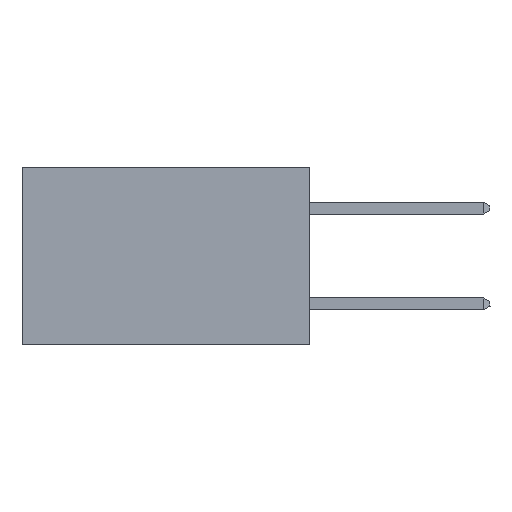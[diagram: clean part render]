
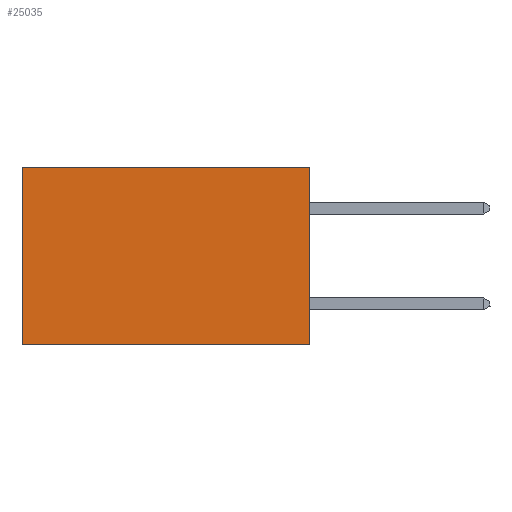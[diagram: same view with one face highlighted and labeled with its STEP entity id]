
A CAD part, left-side view. The second image highlights one B-rep face of the part: STEP entity #25035.
In plain terms, the highlighted planar face has unit normal (-1, 0, 0).
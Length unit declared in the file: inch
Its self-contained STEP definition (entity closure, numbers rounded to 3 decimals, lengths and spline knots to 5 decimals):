
#95 = EDGE_CURVE ( 'NONE', #11923, #24437, #12233, .T. ) ;
#900 = DIRECTION ( 'NONE',  ( 0., 1., 0. ) ) ;
#1596 = DIRECTION ( 'NONE',  ( 0., 0., -1. ) ) ;
#2144 = VECTOR ( 'NONE', #900, 39.37008 ) ;
#4816 = EDGE_CURVE ( 'NONE', #11923, #17204, #19692, .T. ) ;
#5724 = CARTESIAN_POINT ( 'NONE',  ( 0.2875, 0., 0. ) ) ;
#6483 = CARTESIAN_POINT ( 'NONE',  ( 0.2875, 0.6, 0. ) ) ;
#7051 = CARTESIAN_POINT ( 'NONE',  ( 0.2875, 0.6, 0. ) ) ;
#8110 = VECTOR ( 'NONE', #15023, 39.37008 ) ;
#8834 = VECTOR ( 'NONE', #14239, 39.37008 ) ;
#10736 = CARTESIAN_POINT ( 'NONE',  ( 0.2875, 0., 0. ) ) ;
#11923 = VERTEX_POINT ( 'NONE', #12074 ) ;
#12074 = CARTESIAN_POINT ( 'NONE',  ( 0.2875, 0., 0. ) ) ;
#12233 = LINE ( 'NONE', #5724, #8110 ) ;
#13004 = DIRECTION ( 'NONE',  ( 1., 0., 0. ) ) ;
#13359 = EDGE_CURVE ( 'NONE', #17204, #30338, #27809, .T. ) ;
#13988 = ORIENTED_EDGE ( 'NONE', *, *, #95, .F. ) ;
#14239 = DIRECTION ( 'NONE',  ( 0., 0., -1. ) ) ;
#14667 = EDGE_CURVE ( 'NONE', #24437, #30338, #15170, .T. ) ;
#15023 = DIRECTION ( 'NONE',  ( 0., 0., -1. ) ) ;
#15170 = LINE ( 'NONE', #23487, #19261 ) ;
#17100 = CARTESIAN_POINT ( 'NONE',  ( 0.2875, 0.6, -0.37 ) ) ;
#17204 = VERTEX_POINT ( 'NONE', #6483 ) ;
#18708 = ORIENTED_EDGE ( 'NONE', *, *, #4816, .T. ) ;
#19261 = VECTOR ( 'NONE', #25589, 39.37008 ) ;
#19692 = LINE ( 'NONE', #10736, #2144 ) ;
#20049 = CARTESIAN_POINT ( 'NONE',  ( 0.2875, 0., 0. ) ) ;
#21058 = AXIS2_PLACEMENT_3D ( 'NONE', #20049, #13004, #1596 ) ;
#22108 = PLANE ( 'NONE',  #21058 ) ;
#23107 = EDGE_LOOP ( 'NONE', ( #28930, #25601, #13988, #18708 ) ) ;
#23365 = CARTESIAN_POINT ( 'NONE',  ( 0.2875, 0., -0.37 ) ) ;
#23487 = CARTESIAN_POINT ( 'NONE',  ( 0.2875, 0., -0.37 ) ) ;
#24437 = VERTEX_POINT ( 'NONE', #23365 ) ;
#25035 = ADVANCED_FACE ( 'NONE', ( #26280 ), #22108, .F. ) ;
#25589 = DIRECTION ( 'NONE',  ( 0., 1., 0. ) ) ;
#25601 = ORIENTED_EDGE ( 'NONE', *, *, #14667, .F. ) ;
#26280 = FACE_OUTER_BOUND ( 'NONE', #23107, .T. ) ;
#27809 = LINE ( 'NONE', #7051, #8834 ) ;
#28930 = ORIENTED_EDGE ( 'NONE', *, *, #13359, .T. ) ;
#30338 = VERTEX_POINT ( 'NONE', #17100 ) ;
